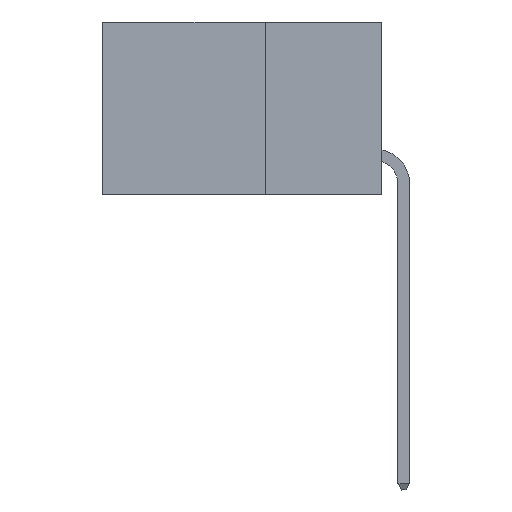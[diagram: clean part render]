
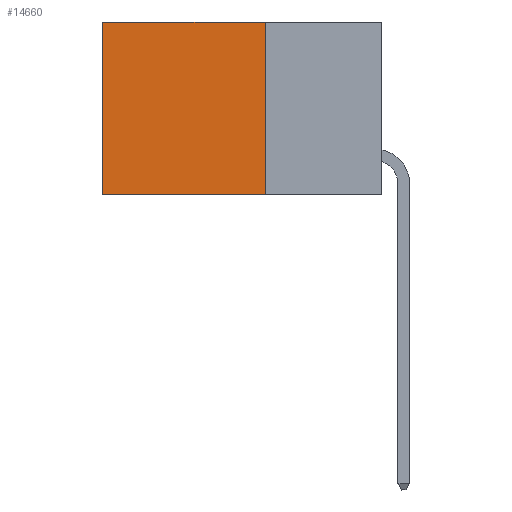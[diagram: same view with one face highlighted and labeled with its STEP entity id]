
A CAD part, left-side view. The second image highlights one B-rep face of the part: STEP entity #14660.
In plain terms, the highlighted planar face has unit normal (-1, 0, 0).
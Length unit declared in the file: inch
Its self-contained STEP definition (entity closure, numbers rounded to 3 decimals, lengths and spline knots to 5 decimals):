
#52 = DIRECTION ( 'NONE',  ( 0., 1., 0. ) ) ;
#85 = CARTESIAN_POINT ( 'NONE',  ( 0.2875, 0.25, -0.37 ) ) ;
#176 = VECTOR ( 'NONE', #2925, 39.37008 ) ;
#525 = VERTEX_POINT ( 'NONE', #7268 ) ;
#698 = EDGE_CURVE ( 'NONE', #4235, #11836, #5260, .T. ) ;
#828 = CARTESIAN_POINT ( 'NONE',  ( 0.2875, 0.25, 0. ) ) ;
#989 = ORIENTED_EDGE ( 'NONE', *, *, #7644, .F. ) ;
#2925 = DIRECTION ( 'NONE',  ( 0., 0., -1. ) ) ;
#3819 = VERTEX_POINT ( 'NONE', #85 ) ;
#3962 = VECTOR ( 'NONE', #16524, 39.37008 ) ;
#4032 = LINE ( 'NONE', #828, #15161 ) ;
#4192 = CARTESIAN_POINT ( 'NONE',  ( 0.2875, 0.25, 0. ) ) ;
#4235 = VERTEX_POINT ( 'NONE', #7277 ) ;
#4260 = DIRECTION ( 'NONE',  ( 0., 0., -1. ) ) ;
#5260 = LINE ( 'NONE', #15422, #176 ) ;
#6599 = ORIENTED_EDGE ( 'NONE', *, *, #698, .T. ) ;
#6986 = CARTESIAN_POINT ( 'NONE',  ( 0.2875, 0.25, 0. ) ) ;
#7221 = LINE ( 'NONE', #8104, #3962 ) ;
#7268 = CARTESIAN_POINT ( 'NONE',  ( 0.2875, 0.25, 0. ) ) ;
#7277 = CARTESIAN_POINT ( 'NONE',  ( 0.2875, 0.6, 0. ) ) ;
#7644 = EDGE_CURVE ( 'NONE', #3819, #11836, #7221, .T. ) ;
#7715 = DIRECTION ( 'NONE',  ( 0., 0., -1. ) ) ;
#8104 = CARTESIAN_POINT ( 'NONE',  ( 0.2875, 0.25, -0.37 ) ) ;
#8518 = PLANE ( 'NONE',  #13893 ) ;
#8655 = ORIENTED_EDGE ( 'NONE', *, *, #10938, .F. ) ;
#10864 = FACE_OUTER_BOUND ( 'NONE', #12341, .T. ) ;
#10884 = CARTESIAN_POINT ( 'NONE',  ( 0.2875, 0.6, -0.37 ) ) ;
#10938 = EDGE_CURVE ( 'NONE', #525, #3819, #4032, .T. ) ;
#11836 = VERTEX_POINT ( 'NONE', #10884 ) ;
#12341 = EDGE_LOOP ( 'NONE', ( #6599, #989, #8655, #17611 ) ) ;
#13893 = AXIS2_PLACEMENT_3D ( 'NONE', #4192, #15344, #4260 ) ;
#14660 = ADVANCED_FACE ( 'NONE', ( #10864 ), #8518, .F. ) ;
#14666 = EDGE_CURVE ( 'NONE', #525, #4235, #15694, .T. ) ;
#15161 = VECTOR ( 'NONE', #7715, 39.37008 ) ;
#15344 = DIRECTION ( 'NONE',  ( 1., 0., 0. ) ) ;
#15422 = CARTESIAN_POINT ( 'NONE',  ( 0.2875, 0.6, 0. ) ) ;
#15465 = VECTOR ( 'NONE', #52, 39.37008 ) ;
#15694 = LINE ( 'NONE', #6986, #15465 ) ;
#16524 = DIRECTION ( 'NONE',  ( 0., 1., 0. ) ) ;
#17611 = ORIENTED_EDGE ( 'NONE', *, *, #14666, .T. ) ;
